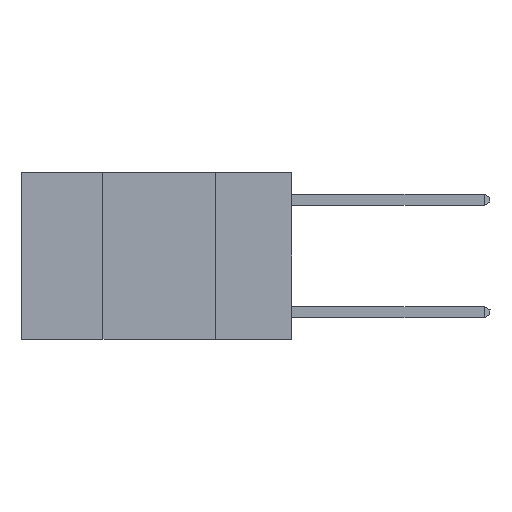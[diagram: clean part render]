
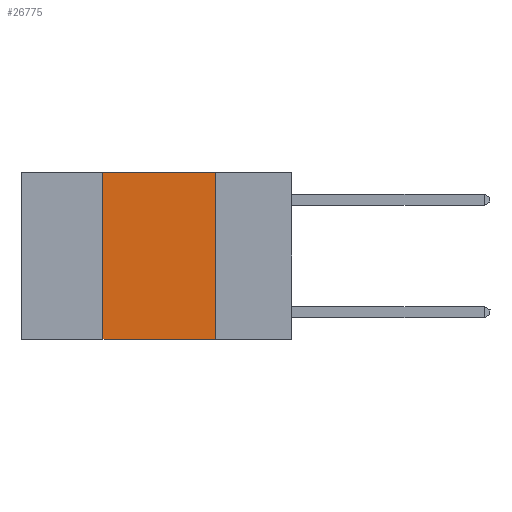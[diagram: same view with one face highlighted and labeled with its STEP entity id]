
A CAD part, left-side view. The second image highlights one B-rep face of the part: STEP entity #26775.
In plain terms, the highlighted planar face has unit normal (-1, 0, 0).
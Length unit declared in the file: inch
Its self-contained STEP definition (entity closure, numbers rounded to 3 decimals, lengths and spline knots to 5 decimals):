
#2 = DIRECTION ( 'NONE',  ( 0., 0., -1. ) ) ;
#591 = CARTESIAN_POINT ( 'NONE',  ( 0., 0.42, 0. ) ) ;
#2267 = AXIS2_PLACEMENT_3D ( 'NONE', #26636, #14681, #2 ) ;
#2513 = ORIENTED_EDGE ( 'NONE', *, *, #6961, .F. ) ;
#3067 = DIRECTION ( 'NONE',  ( 0., 0., 1. ) ) ;
#3257 = EDGE_LOOP ( 'NONE', ( #2513, #22591, #29581, #27177 ) ) ;
#3328 = DIRECTION ( 'NONE',  ( 0., -1., 0. ) ) ;
#4336 = CARTESIAN_POINT ( 'NONE',  ( 0., 0.17, 0. ) ) ;
#6590 = EDGE_CURVE ( 'NONE', #9278, #8201, #16455, .T. ) ;
#6961 = EDGE_CURVE ( 'NONE', #7683, #27657, #30553, .T. ) ;
#6975 = VECTOR ( 'NONE', #26006, 39.37008 ) ;
#7683 = VERTEX_POINT ( 'NONE', #23892 ) ;
#7964 = CARTESIAN_POINT ( 'NONE',  ( 0., 0.42, -0.37 ) ) ;
#8201 = VERTEX_POINT ( 'NONE', #23340 ) ;
#9278 = VERTEX_POINT ( 'NONE', #7964 ) ;
#10455 = VECTOR ( 'NONE', #3328, 39.37008 ) ;
#11426 = EDGE_CURVE ( 'NONE', #8201, #7683, #16947, .T. ) ;
#13457 = LINE ( 'NONE', #28436, #6975 ) ;
#14681 = DIRECTION ( 'NONE',  ( 1., 0., 0. ) ) ;
#16455 = LINE ( 'NONE', #591, #23571 ) ;
#16947 = LINE ( 'NONE', #20293, #10455 ) ;
#19581 = FACE_OUTER_BOUND ( 'NONE', #3257, .T. ) ;
#20293 = CARTESIAN_POINT ( 'NONE',  ( 0., 0.6, 0. ) ) ;
#22591 = ORIENTED_EDGE ( 'NONE', *, *, #11426, .F. ) ;
#23340 = CARTESIAN_POINT ( 'NONE',  ( 0., 0.42, 0. ) ) ;
#23571 = VECTOR ( 'NONE', #3067, 39.37008 ) ;
#23892 = CARTESIAN_POINT ( 'NONE',  ( 0., 0.17, 0. ) ) ;
#25806 = VECTOR ( 'NONE', #28373, 39.37008 ) ;
#26006 = DIRECTION ( 'NONE',  ( 0., -1., 0. ) ) ;
#26636 = CARTESIAN_POINT ( 'NONE',  ( 0., 0.6, 0. ) ) ;
#26775 = ADVANCED_FACE ( 'NONE', ( #19581 ), #28964, .F. ) ;
#27177 = ORIENTED_EDGE ( 'NONE', *, *, #28786, .T. ) ;
#27386 = CARTESIAN_POINT ( 'NONE',  ( 0., 0.17, -0.37 ) ) ;
#27657 = VERTEX_POINT ( 'NONE', #27386 ) ;
#28373 = DIRECTION ( 'NONE',  ( 0., 0., -1. ) ) ;
#28436 = CARTESIAN_POINT ( 'NONE',  ( 0., 0.6, -0.37 ) ) ;
#28786 = EDGE_CURVE ( 'NONE', #9278, #27657, #13457, .T. ) ;
#28964 = PLANE ( 'NONE',  #2267 ) ;
#29581 = ORIENTED_EDGE ( 'NONE', *, *, #6590, .F. ) ;
#30553 = LINE ( 'NONE', #4336, #25806 ) ;
